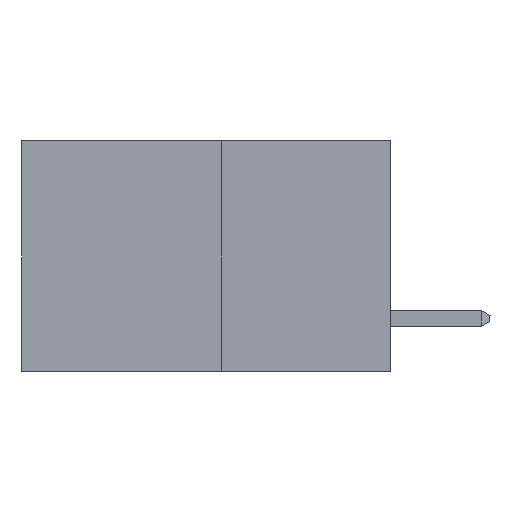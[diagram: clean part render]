
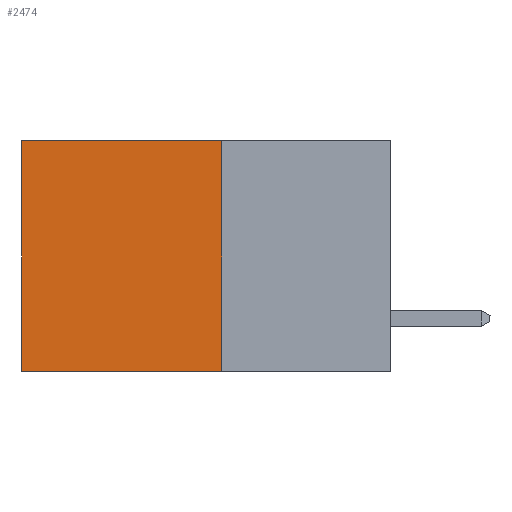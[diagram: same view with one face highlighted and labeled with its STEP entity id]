
A CAD part, left-side view. The second image highlights one B-rep face of the part: STEP entity #2474.
In plain terms, the highlighted planar face has unit normal (-1, 0, 0).
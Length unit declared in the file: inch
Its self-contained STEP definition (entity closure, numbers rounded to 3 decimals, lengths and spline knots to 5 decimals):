
#46 = FACE_OUTER_BOUND ( 'NONE', #11974, .T. ) ;
#132 = ORIENTED_EDGE ( 'NONE', *, *, #3987, .T. ) ;
#163 = VERTEX_POINT ( 'NONE', #6349 ) ;
#1503 = ORIENTED_EDGE ( 'NONE', *, *, #4822, .F. ) ;
#2073 = ORIENTED_EDGE ( 'NONE', *, *, #3596, .T. ) ;
#2277 = LINE ( 'NONE', #9172, #11406 ) ;
#2474 = ADVANCED_FACE ( 'NONE', ( #46 ), #10882, .F. ) ;
#2600 = ORIENTED_EDGE ( 'NONE', *, *, #8989, .F. ) ;
#3224 = VERTEX_POINT ( 'NONE', #6068 ) ;
#3596 = EDGE_CURVE ( 'NONE', #163, #3224, #2277, .T. ) ;
#3987 = EDGE_CURVE ( 'NONE', #5273, #163, #7626, .T. ) ;
#4590 = CARTESIAN_POINT ( 'NONE',  ( 0.277, 0.27, -0.37 ) ) ;
#4822 = EDGE_CURVE ( 'NONE', #5273, #10154, #12438, .T. ) ;
#5273 = VERTEX_POINT ( 'NONE', #6815 ) ;
#6068 = CARTESIAN_POINT ( 'NONE',  ( 0.277, 0.59, -0.37 ) ) ;
#6349 = CARTESIAN_POINT ( 'NONE',  ( 0.277, 0.59, 0. ) ) ;
#6815 = CARTESIAN_POINT ( 'NONE',  ( 0.277, 0.27, 0. ) ) ;
#7626 = LINE ( 'NONE', #14909, #13316 ) ;
#8989 = EDGE_CURVE ( 'NONE', #10154, #3224, #13170, .T. ) ;
#9172 = CARTESIAN_POINT ( 'NONE',  ( 0.277, 0.59, -0.37 ) ) ;
#9612 = DIRECTION ( 'NONE',  ( 0., 0., -1. ) ) ;
#10011 = CARTESIAN_POINT ( 'NONE',  ( 0.277, 0.27, -0.37 ) ) ;
#10091 = AXIS2_PLACEMENT_3D ( 'NONE', #4590, #10830, #13100 ) ;
#10154 = VERTEX_POINT ( 'NONE', #15079 ) ;
#10830 = DIRECTION ( 'NONE',  ( 1., 0., 0. ) ) ;
#10882 = PLANE ( 'NONE',  #10091 ) ;
#11179 = DIRECTION ( 'NONE',  ( 0., 1., 0. ) ) ;
#11406 = VECTOR ( 'NONE', #9612, 39.37008 ) ;
#11408 = VECTOR ( 'NONE', #11179, 39.37008 ) ;
#11912 = CARTESIAN_POINT ( 'NONE',  ( 0.277, 0.27, -0.37 ) ) ;
#11974 = EDGE_LOOP ( 'NONE', ( #2073, #2600, #1503, #132 ) ) ;
#12092 = VECTOR ( 'NONE', #12614, 39.37008 ) ;
#12438 = LINE ( 'NONE', #11912, #12092 ) ;
#12614 = DIRECTION ( 'NONE',  ( 0., 0., -1. ) ) ;
#13100 = DIRECTION ( 'NONE',  ( 0., 0., -1. ) ) ;
#13170 = LINE ( 'NONE', #10011, #11408 ) ;
#13316 = VECTOR ( 'NONE', #14725, 39.37008 ) ;
#14725 = DIRECTION ( 'NONE',  ( 0., 1., 0. ) ) ;
#14909 = CARTESIAN_POINT ( 'NONE',  ( 0.277, 0.27, 0. ) ) ;
#15079 = CARTESIAN_POINT ( 'NONE',  ( 0.277, 0.27, -0.37 ) ) ;
